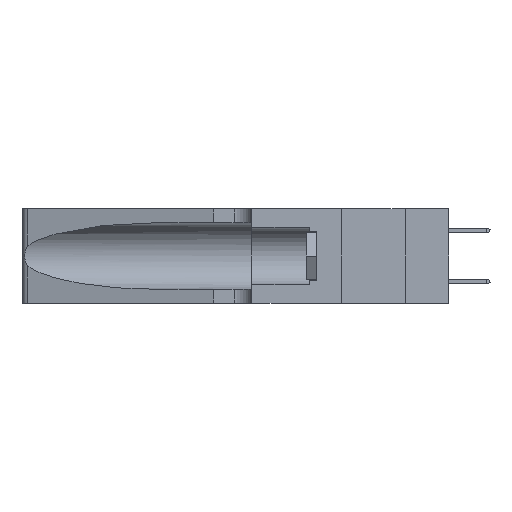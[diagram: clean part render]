
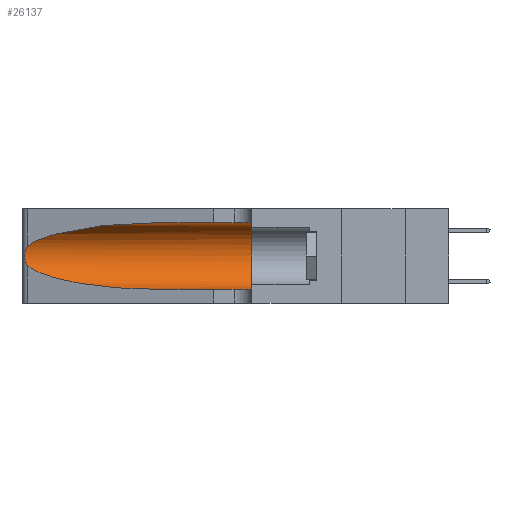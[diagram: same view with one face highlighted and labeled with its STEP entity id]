
A CAD part, left-side view. The second image highlights one B-rep face of the part: STEP entity #26137.
In plain terms, the highlighted cylindrical face has radius 3.308 mm (diameter 6.617 mm), a partial arc.
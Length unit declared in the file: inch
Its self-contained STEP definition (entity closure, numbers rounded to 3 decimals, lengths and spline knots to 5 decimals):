
#151 = EDGE_CURVE ( 'NONE', #23001, #9199, #10745, .T. ) ;
#1680 = DIRECTION ( 'NONE',  ( 0., 0., 1. ) ) ;
#1717 = LINE ( 'NONE', #23846, #6781 ) ;
#2115 = CARTESIAN_POINT ( 'NONE',  ( 0.26018, 1.23835, 0.19895 ) ) ;
#2804 = CARTESIAN_POINT ( 'NONE',  ( 0.1305, 1.61858, 0.05475 ) ) ;
#4275 = CARTESIAN_POINT ( 'NONE',  ( 0.26075, 1.23896, 0.178 ) ) ;
#4578 = CARTESIAN_POINT ( 'NONE',  ( 0.2373, 1.15595, 0.08982 ) ) ;
#4632 = ORIENTED_EDGE ( 'NONE', *, *, #10612, .F. ) ;
#5044 = ORIENTED_EDGE ( 'NONE', *, *, #14469, .T. ) ;
#5071 = CARTESIAN_POINT ( 'NONE',  ( 0.1305, 1.61858, 0.185 ) ) ;
#6451 = CARTESIAN_POINT ( 'NONE',  ( 0.25856, 1.23593, 0.16098 ) ) ;
#6563 = CARTESIAN_POINT ( 'NONE',  ( 0.25487, 1.22718, 0.22369 ) ) ;
#6776 = CARTESIAN_POINT ( 'NONE',  ( 0.18966, 0.96281, 0.05475 ) ) ;
#6781 = VECTOR ( 'NONE', #25933, 39.37008 ) ;
#6830 = VERTEX_POINT ( 'NONE', #16369 ) ;
#6958 = CARTESIAN_POINT ( 'NONE',  ( 0.1305, 0.72297, 0.31525 ) ) ;
#7535 = AXIS2_PLACEMENT_3D ( 'NONE', #5071, #13700, #24170 ) ;
#8469 = CARTESIAN_POINT ( 'NONE',  ( 0.25555, 1.22994, 0.2215 ) ) ;
#8555 = CARTESIAN_POINT ( 'NONE',  ( 0.25487, 1.22718, 0.22369 ) ) ;
#8643 = CARTESIAN_POINT ( 'NONE',  ( 0.25639, 1.23186, 0.15144 ) ) ;
#8861 = CARTESIAN_POINT ( 'NONE',  ( 0.25487, 1.22718, 0.14631 ) ) ;
#9199 = VERTEX_POINT ( 'NONE', #14341 ) ;
#9331 = CARTESIAN_POINT ( 'NONE',  ( 0.1305, 0.35, 0.05475 ) ) ;
#9683 = FACE_OUTER_BOUND ( 'NONE', #11174, .T. ) ;
#9787 = CARTESIAN_POINT ( 'NONE',  ( 0.18966, 0.96281, 0.31525 ) ) ;
#9979 = ORIENTED_EDGE ( 'NONE', *, *, #27051, .T. ) ;
#10402 = AXIS2_PLACEMENT_3D ( 'NONE', #27108, #14550, #1680 ) ;
#10612 = EDGE_CURVE ( 'NONE', #6830, #21103, #12892, .T. ) ;
#10745 =( BOUNDED_CURVE ( )  B_SPLINE_CURVE ( 3, ( #25385, #9787, #17868, #6563 ),
 .UNSPECIFIED., .F., .F. ) 
 B_SPLINE_CURVE_WITH_KNOTS ( ( 4, 4 ),
 ( 1.5708, 2.84003 ),
 .UNSPECIFIED. ) 
 CURVE ( )  GEOMETRIC_REPRESENTATION_ITEM ( )  RATIONAL_B_SPLINE_CURVE ( ( 1., 0.87, 0.87, 1. ) ) 
 REPRESENTATION_ITEM ( '' )  );
#10809 = CARTESIAN_POINT ( 'NONE',  ( 0.25487, 1.22718, 0.14631 ) ) ;
#11174 = EDGE_LOOP ( 'NONE', ( #25136, #17939, #9979, #5044, #4632, #16409 ) ) ;
#11595 =( BOUNDED_CURVE ( )  B_SPLINE_CURVE ( 3, ( #8861, #4578, #6776, #21614 ),
 .UNSPECIFIED., .F., .T. ) 
 B_SPLINE_CURVE_WITH_KNOTS ( ( 4, 4 ),
 ( 3.44316, 4.71239 ),
 .UNSPECIFIED. ) 
 CURVE ( )  GEOMETRIC_REPRESENTATION_ITEM ( )  RATIONAL_B_SPLINE_CURVE ( ( 1., 0.87, 0.87, 1. ) ) 
 REPRESENTATION_ITEM ( '' )  );
#12788 = VERTEX_POINT ( 'NONE', #22411 ) ;
#12852 = CARTESIAN_POINT ( 'NONE',  ( 0.25639, 1.23184, 0.21858 ) ) ;
#12892 = CIRCLE ( 'NONE', #10402, 0.13025 ) ;
#13700 = DIRECTION ( 'NONE',  ( 0., -1., 0. ) ) ;
#14341 = CARTESIAN_POINT ( 'NONE',  ( 0.25487, 1.22718, 0.22369 ) ) ;
#14469 = EDGE_CURVE ( 'NONE', #12788, #21103, #14706, .T. ) ;
#14550 = DIRECTION ( 'NONE',  ( 0., 1., 0. ) ) ;
#14706 = LINE ( 'NONE', #2804, #19630 ) ;
#14960 = CARTESIAN_POINT ( 'NONE',  ( 0.25854, 1.2359, 0.20912 ) ) ;
#15648 = DIRECTION ( 'NONE',  ( 0., -1., 0. ) ) ;
#16369 = CARTESIAN_POINT ( 'NONE',  ( 0.1305, 0.35, 0.31525 ) ) ;
#16409 = ORIENTED_EDGE ( 'NONE', *, *, #23430, .F. ) ;
#17097 = CARTESIAN_POINT ( 'NONE',  ( 0.26075, 1.23896, 0.19203 ) ) ;
#17868 = CARTESIAN_POINT ( 'NONE',  ( 0.2373, 1.15595, 0.28018 ) ) ;
#17939 = ORIENTED_EDGE ( 'NONE', *, *, #21494, .T. ) ;
#18466 = CARTESIAN_POINT ( 'NONE',  ( 0.25487, 1.22718, 0.14631 ) ) ;
#18721 = VERTEX_POINT ( 'NONE', #18466 ) ;
#19192 = CARTESIAN_POINT ( 'NONE',  ( 0.26017, 1.23833, 0.17102 ) ) ;
#19630 = VECTOR ( 'NONE', #15648, 39.37008 ) ;
#21103 = VERTEX_POINT ( 'NONE', #9331 ) ;
#21319 = CARTESIAN_POINT ( 'NONE',  ( 0.25789, 1.23486, 0.15765 ) ) ;
#21494 = EDGE_CURVE ( 'NONE', #9199, #18721, #26246, .T. ) ;
#21614 = CARTESIAN_POINT ( 'NONE',  ( 0.1305, 0.72297, 0.05475 ) ) ;
#22411 = CARTESIAN_POINT ( 'NONE',  ( 0.1305, 0.72297, 0.05475 ) ) ;
#23001 = VERTEX_POINT ( 'NONE', #6958 ) ;
#23429 = CARTESIAN_POINT ( 'NONE',  ( 0.25555, 1.22993, 0.14849 ) ) ;
#23430 = EDGE_CURVE ( 'NONE', #23001, #6830, #1717, .T. ) ;
#23846 = CARTESIAN_POINT ( 'NONE',  ( 0.1305, 1.61858, 0.31525 ) ) ;
#24170 = DIRECTION ( 'NONE',  ( 0., 0., -1. ) ) ;
#24502 = CYLINDRICAL_SURFACE ( 'NONE', #7535, 0.13025 ) ;
#25136 = ORIENTED_EDGE ( 'NONE', *, *, #151, .T. ) ;
#25385 = CARTESIAN_POINT ( 'NONE',  ( 0.1305, 0.72297, 0.31525 ) ) ;
#25933 = DIRECTION ( 'NONE',  ( 0., -1., 0. ) ) ;
#26137 = ADVANCED_FACE ( 'NONE', ( #9683 ), #24502, .F. ) ;
#26246 = B_SPLINE_CURVE_WITH_KNOTS ( 'NONE', 3,
 ( #8555, #8469, #12852, #27523, #14960, #2115, #17097, #4275, #19192, #6451, #21319, #8643, #23429, #10809 ),
 .UNSPECIFIED., .F., .F.,
 ( 4, 2, 2, 2, 2, 2, 4 ),
 ( 0., 0.00027, 0.00053, 0.00107, 0.0016, 0.00187, 0.00214 ),
 .UNSPECIFIED. ) ;
#27051 = EDGE_CURVE ( 'NONE', #18721, #12788, #11595, .T. ) ;
#27108 = CARTESIAN_POINT ( 'NONE',  ( 0.1305, 0.35, 0.185 ) ) ;
#27523 = CARTESIAN_POINT ( 'NONE',  ( 0.25787, 1.23484, 0.2124 ) ) ;
